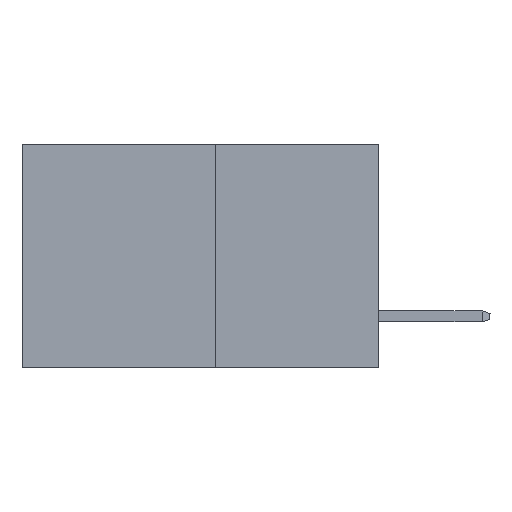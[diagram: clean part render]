
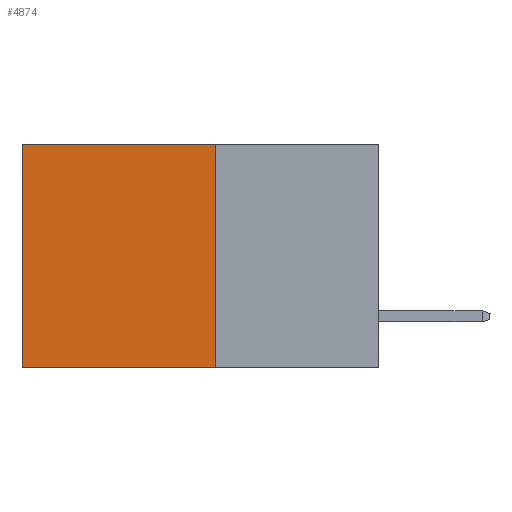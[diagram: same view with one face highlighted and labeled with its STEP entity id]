
A CAD part, left-side view. The second image highlights one B-rep face of the part: STEP entity #4874.
In plain terms, the highlighted planar face has unit normal (-1, 0, 0).
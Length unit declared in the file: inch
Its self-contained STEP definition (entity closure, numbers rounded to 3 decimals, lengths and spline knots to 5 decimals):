
#217 = CARTESIAN_POINT ( 'NONE',  ( 0.277, 0.59, -0.37 ) ) ;
#1674 = AXIS2_PLACEMENT_3D ( 'NONE', #10300, #3756, #27263 ) ;
#1983 = ORIENTED_EDGE ( 'NONE', *, *, #8106, .F. ) ;
#2377 = CARTESIAN_POINT ( 'NONE',  ( 0.277, 0.59, -0.37 ) ) ;
#3088 = LINE ( 'NONE', #217, #24515 ) ;
#3756 = DIRECTION ( 'NONE',  ( 1., 0., 0. ) ) ;
#4473 = CARTESIAN_POINT ( 'NONE',  ( 0.277, 0.27, 0. ) ) ;
#4735 = FACE_OUTER_BOUND ( 'NONE', #13156, .T. ) ;
#4874 = ADVANCED_FACE ( 'NONE', ( #4735 ), #10161, .F. ) ;
#5423 = DIRECTION ( 'NONE',  ( 0., 0., -1. ) ) ;
#5516 = CARTESIAN_POINT ( 'NONE',  ( 0.277, 0.27, -0.37 ) ) ;
#6189 = VECTOR ( 'NONE', #23593, 39.37008 ) ;
#7152 = VERTEX_POINT ( 'NONE', #20034 ) ;
#8106 = EDGE_CURVE ( 'NONE', #7152, #8939, #11497, .T. ) ;
#8939 = VERTEX_POINT ( 'NONE', #2377 ) ;
#9267 = ORIENTED_EDGE ( 'NONE', *, *, #19256, .T. ) ;
#9619 = LINE ( 'NONE', #4473, #15690 ) ;
#10161 = PLANE ( 'NONE',  #1674 ) ;
#10300 = CARTESIAN_POINT ( 'NONE',  ( 0.277, 0.27, -0.37 ) ) ;
#11097 = VECTOR ( 'NONE', #11601, 39.37008 ) ;
#11497 = LINE ( 'NONE', #5516, #6189 ) ;
#11601 = DIRECTION ( 'NONE',  ( 0., 0., -1. ) ) ;
#13142 = EDGE_CURVE ( 'NONE', #25655, #25205, #9619, .T. ) ;
#13156 = EDGE_LOOP ( 'NONE', ( #9267, #1983, #14218, #29565 ) ) ;
#14218 = ORIENTED_EDGE ( 'NONE', *, *, #31158, .F. ) ;
#15575 = CARTESIAN_POINT ( 'NONE',  ( 0.277, 0.27, 0. ) ) ;
#15690 = VECTOR ( 'NONE', #30297, 39.37008 ) ;
#19256 = EDGE_CURVE ( 'NONE', #25205, #8939, #3088, .T. ) ;
#20034 = CARTESIAN_POINT ( 'NONE',  ( 0.277, 0.27, -0.37 ) ) ;
#23593 = DIRECTION ( 'NONE',  ( 0., 1., 0. ) ) ;
#23975 = LINE ( 'NONE', #24399, #11097 ) ;
#24399 = CARTESIAN_POINT ( 'NONE',  ( 0.277, 0.27, -0.37 ) ) ;
#24515 = VECTOR ( 'NONE', #5423, 39.37008 ) ;
#25205 = VERTEX_POINT ( 'NONE', #26715 ) ;
#25655 = VERTEX_POINT ( 'NONE', #15575 ) ;
#26715 = CARTESIAN_POINT ( 'NONE',  ( 0.277, 0.59, 0. ) ) ;
#27263 = DIRECTION ( 'NONE',  ( 0., 0., -1. ) ) ;
#29565 = ORIENTED_EDGE ( 'NONE', *, *, #13142, .T. ) ;
#30297 = DIRECTION ( 'NONE',  ( 0., 1., 0. ) ) ;
#31158 = EDGE_CURVE ( 'NONE', #25655, #7152, #23975, .T. ) ;
